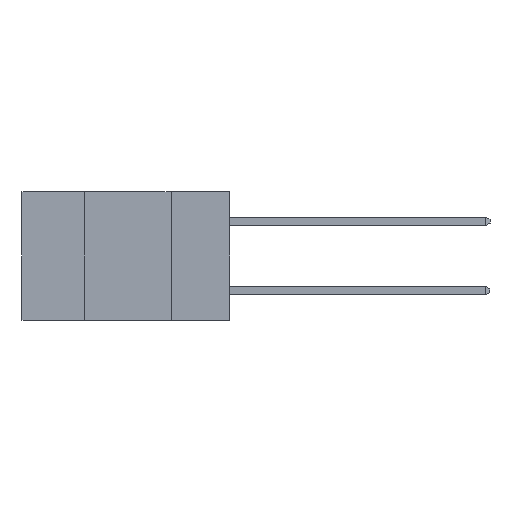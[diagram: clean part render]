
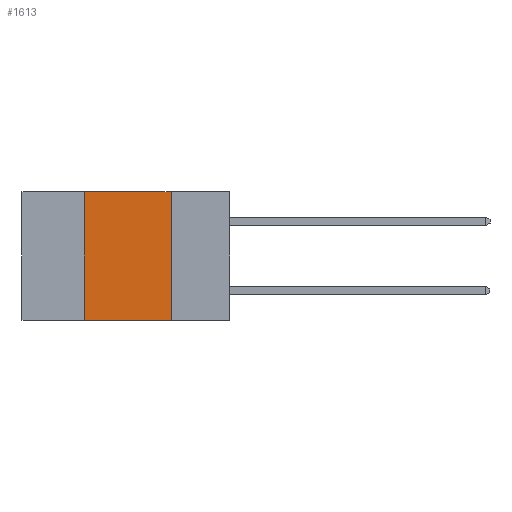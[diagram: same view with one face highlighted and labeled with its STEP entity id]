
A CAD part, left-side view. The second image highlights one B-rep face of the part: STEP entity #1613.
In plain terms, the highlighted planar face has unit normal (-1, 0, 0).
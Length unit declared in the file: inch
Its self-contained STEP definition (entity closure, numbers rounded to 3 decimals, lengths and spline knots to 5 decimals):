
#169 = LINE ( 'NONE', #12787, #8267 ) ;
#305 = EDGE_CURVE ( 'NONE', #6333, #9993, #3099, .T. ) ;
#561 = DIRECTION ( 'NONE',  ( 0., -1., 0. ) ) ;
#1591 = CARTESIAN_POINT ( 'NONE',  ( 0., 0.42, 0. ) ) ;
#1609 = DIRECTION ( 'NONE',  ( 0., 0., 1. ) ) ;
#1613 = ADVANCED_FACE ( 'NONE', ( #11079 ), #5729, .F. ) ;
#3099 = LINE ( 'NONE', #3244, #3446 ) ;
#3244 = CARTESIAN_POINT ( 'NONE',  ( 0., 0.17, 0. ) ) ;
#3247 = EDGE_CURVE ( 'NONE', #8896, #12892, #10104, .T. ) ;
#3446 = VECTOR ( 'NONE', #9086, 39.37008 ) ;
#4212 = LINE ( 'NONE', #4914, #11945 ) ;
#4914 = CARTESIAN_POINT ( 'NONE',  ( 0., 0.6, 0. ) ) ;
#4994 = CARTESIAN_POINT ( 'NONE',  ( 0., 0.17, 0. ) ) ;
#5041 = CARTESIAN_POINT ( 'NONE',  ( 0., 0.17, -0.37 ) ) ;
#5212 = ORIENTED_EDGE ( 'NONE', *, *, #7598, .F. ) ;
#5632 = ORIENTED_EDGE ( 'NONE', *, *, #3247, .F. ) ;
#5637 = EDGE_LOOP ( 'NONE', ( #11039, #5212, #5632, #6636 ) ) ;
#5729 = PLANE ( 'NONE',  #11421 ) ;
#6333 = VERTEX_POINT ( 'NONE', #4994 ) ;
#6636 = ORIENTED_EDGE ( 'NONE', *, *, #9836, .T. ) ;
#7546 = DIRECTION ( 'NONE',  ( 0., 0., -1. ) ) ;
#7562 = DIRECTION ( 'NONE',  ( 1., 0., 0. ) ) ;
#7598 = EDGE_CURVE ( 'NONE', #12892, #6333, #4212, .T. ) ;
#7852 = CARTESIAN_POINT ( 'NONE',  ( 0., 0.6, 0. ) ) ;
#7888 = DIRECTION ( 'NONE',  ( 0., -1., 0. ) ) ;
#8267 = VECTOR ( 'NONE', #561, 39.37008 ) ;
#8896 = VERTEX_POINT ( 'NONE', #11393 ) ;
#9086 = DIRECTION ( 'NONE',  ( 0., 0., -1. ) ) ;
#9836 = EDGE_CURVE ( 'NONE', #8896, #9993, #169, .T. ) ;
#9993 = VERTEX_POINT ( 'NONE', #5041 ) ;
#10104 = LINE ( 'NONE', #1591, #12358 ) ;
#11039 = ORIENTED_EDGE ( 'NONE', *, *, #305, .F. ) ;
#11079 = FACE_OUTER_BOUND ( 'NONE', #5637, .T. ) ;
#11393 = CARTESIAN_POINT ( 'NONE',  ( 0., 0.42, -0.37 ) ) ;
#11421 = AXIS2_PLACEMENT_3D ( 'NONE', #7852, #7562, #7546 ) ;
#11945 = VECTOR ( 'NONE', #7888, 39.37008 ) ;
#12029 = CARTESIAN_POINT ( 'NONE',  ( 0., 0.42, 0. ) ) ;
#12358 = VECTOR ( 'NONE', #1609, 39.37008 ) ;
#12787 = CARTESIAN_POINT ( 'NONE',  ( 0., 0.6, -0.37 ) ) ;
#12892 = VERTEX_POINT ( 'NONE', #12029 ) ;
